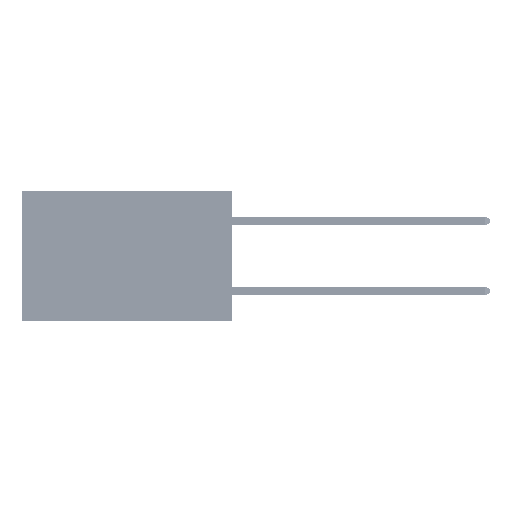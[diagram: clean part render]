
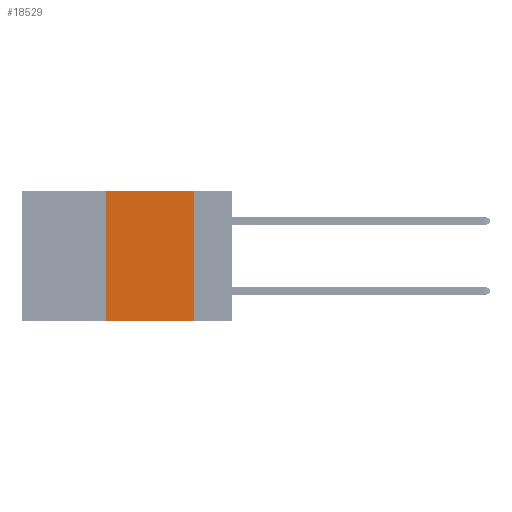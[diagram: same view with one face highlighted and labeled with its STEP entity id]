
A CAD part, left-side view. The second image highlights one B-rep face of the part: STEP entity #18529.
In plain terms, the highlighted planar face has unit normal (-1, 0, 0).
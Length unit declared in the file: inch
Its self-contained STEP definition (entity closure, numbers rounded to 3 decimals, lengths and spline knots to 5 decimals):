
#1307 = VECTOR ( 'NONE', #9337, 39.37008 ) ;
#1455 = LINE ( 'NONE', #45155, #20982 ) ;
#1606 = DIRECTION ( 'NONE',  ( 0., 0., -1. ) ) ;
#2067 = CARTESIAN_POINT ( 'NONE',  ( 0., 0.6, 0. ) ) ;
#5956 = VECTOR ( 'NONE', #12192, 39.37008 ) ;
#6714 = EDGE_CURVE ( 'NONE', #33029, #28136, #7657, .T. ) ;
#7657 = LINE ( 'NONE', #45153, #5956 ) ;
#8483 = CARTESIAN_POINT ( 'NONE',  ( 0., 0.36, 0. ) ) ;
#9122 = DIRECTION ( 'NONE',  ( 0., 0., -1. ) ) ;
#9337 = DIRECTION ( 'NONE',  ( 0., -1., 0. ) ) ;
#10657 = VECTOR ( 'NONE', #15086, 39.37008 ) ;
#12192 = DIRECTION ( 'NONE',  ( 0., -1., 0. ) ) ;
#13328 = CARTESIAN_POINT ( 'NONE',  ( 0., 0.36, -0.37 ) ) ;
#15086 = DIRECTION ( 'NONE',  ( 0., 0., 1. ) ) ;
#18181 = EDGE_LOOP ( 'NONE', ( #33017, #34683, #26756, #27848 ) ) ;
#18529 = ADVANCED_FACE ( 'NONE', ( #21391 ), #46121, .F. ) ;
#19948 = CARTESIAN_POINT ( 'NONE',  ( 0., 0.11, -0.37 ) ) ;
#20767 = EDGE_CURVE ( 'NONE', #33029, #22138, #28362, .T. ) ;
#20828 = LINE ( 'NONE', #45651, #1307 ) ;
#20982 = VECTOR ( 'NONE', #9122, 39.37008 ) ;
#21391 = FACE_OUTER_BOUND ( 'NONE', #18181, .T. ) ;
#22138 = VERTEX_POINT ( 'NONE', #8483 ) ;
#26756 = ORIENTED_EDGE ( 'NONE', *, *, #20767, .F. ) ;
#27848 = ORIENTED_EDGE ( 'NONE', *, *, #6714, .T. ) ;
#28136 = VERTEX_POINT ( 'NONE', #19948 ) ;
#28362 = LINE ( 'NONE', #29017, #10657 ) ;
#28642 = VERTEX_POINT ( 'NONE', #44581 ) ;
#29017 = CARTESIAN_POINT ( 'NONE',  ( 0., 0.36, 0. ) ) ;
#31087 = DIRECTION ( 'NONE',  ( 1., 0., 0. ) ) ;
#33017 = ORIENTED_EDGE ( 'NONE', *, *, #47281, .F. ) ;
#33029 = VERTEX_POINT ( 'NONE', #13328 ) ;
#34683 = ORIENTED_EDGE ( 'NONE', *, *, #44246, .F. ) ;
#44246 = EDGE_CURVE ( 'NONE', #22138, #28642, #20828, .T. ) ;
#44581 = CARTESIAN_POINT ( 'NONE',  ( 0., 0.11, 0. ) ) ;
#45153 = CARTESIAN_POINT ( 'NONE',  ( 0., 0.6, -0.37 ) ) ;
#45155 = CARTESIAN_POINT ( 'NONE',  ( 0., 0.11, 0. ) ) ;
#45282 = AXIS2_PLACEMENT_3D ( 'NONE', #2067, #31087, #1606 ) ;
#45651 = CARTESIAN_POINT ( 'NONE',  ( 0., 0.6, 0. ) ) ;
#46121 = PLANE ( 'NONE',  #45282 ) ;
#47281 = EDGE_CURVE ( 'NONE', #28642, #28136, #1455, .T. ) ;
